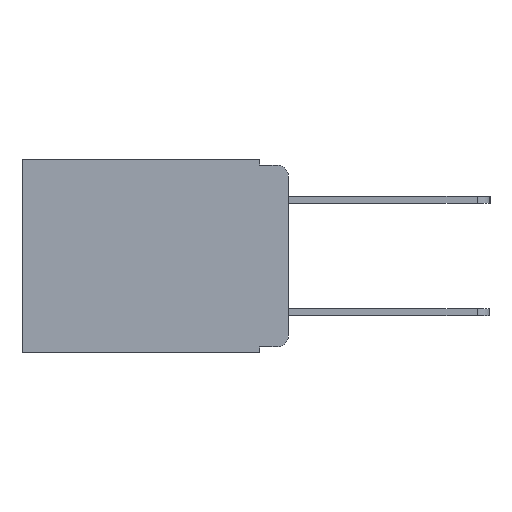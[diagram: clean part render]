
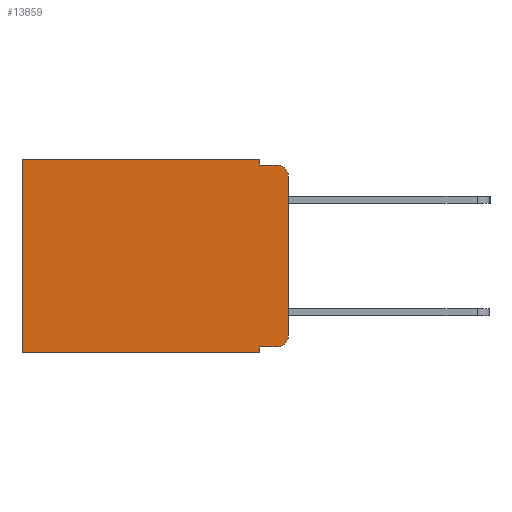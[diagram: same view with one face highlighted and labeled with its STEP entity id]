
A CAD part, left-side view. The second image highlights one B-rep face of the part: STEP entity #13859.
In plain terms, the highlighted planar face has unit normal (-1, 0, 0).
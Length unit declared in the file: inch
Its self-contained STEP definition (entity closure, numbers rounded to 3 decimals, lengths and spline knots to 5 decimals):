
#51 = CARTESIAN_POINT ( 'NONE',  ( 0.298, 0., -0.343 ) ) ;
#1154 = VECTOR ( 'NONE', #17467, 39.37008 ) ;
#1397 = EDGE_LOOP ( 'NONE', ( #1652, #6326, #1983, #3175, #3579, #5256, #9009, #4212, #4299, #4049 ) ) ;
#1432 = EDGE_CURVE ( 'NONE', #13218, #10000, #9390, .T. ) ;
#1652 = ORIENTED_EDGE ( 'NONE', *, *, #7734, .F. ) ;
#1961 = VECTOR ( 'NONE', #17110, 39.37008 ) ;
#1983 = ORIENTED_EDGE ( 'NONE', *, *, #1432, .F. ) ;
#2123 = VECTOR ( 'NONE', #3325, 39.37008 ) ;
#2561 = VECTOR ( 'NONE', #13670, 39.37008 ) ;
#2733 = CIRCLE ( 'NONE', #6456, 0.02 ) ;
#2882 = VECTOR ( 'NONE', #12268, 39.37008 ) ;
#2928 = CARTESIAN_POINT ( 'NONE',  ( 0.298, 0.051, 0. ) ) ;
#3175 = ORIENTED_EDGE ( 'NONE', *, *, #18427, .F. ) ;
#3248 = CARTESIAN_POINT ( 'NONE',  ( 0.298, 0.473, 0. ) ) ;
#3261 = PLANE ( 'NONE',  #17870 ) ;
#3325 = DIRECTION ( 'NONE',  ( 0., 0., -1. ) ) ;
#3501 = DIRECTION ( 'NONE',  ( 0., 0., -1. ) ) ;
#3526 = DIRECTION ( 'NONE',  ( -1., 0., 0. ) ) ;
#3579 = ORIENTED_EDGE ( 'NONE', *, *, #13932, .T. ) ;
#4049 = ORIENTED_EDGE ( 'NONE', *, *, #10074, .T. ) ;
#4212 = ORIENTED_EDGE ( 'NONE', *, *, #13877, .F. ) ;
#4299 = ORIENTED_EDGE ( 'NONE', *, *, #11007, .T. ) ;
#4329 = VERTEX_POINT ( 'NONE', #5411 ) ;
#4592 = EDGE_CURVE ( 'NONE', #17479, #10000, #2733, .T. ) ;
#4647 = CARTESIAN_POINT ( 'NONE',  ( 0.298, 0., -0.03 ) ) ;
#4791 = FACE_OUTER_BOUND ( 'NONE', #1397, .T. ) ;
#5071 = CARTESIAN_POINT ( 'NONE',  ( 0.298, 0.473, 0. ) ) ;
#5256 = ORIENTED_EDGE ( 'NONE', *, *, #15761, .T. ) ;
#5411 = CARTESIAN_POINT ( 'NONE',  ( 0.298, 0.051, -0.333 ) ) ;
#5616 = CARTESIAN_POINT ( 'NONE',  ( 0.298, 0.051, -0.333 ) ) ;
#6011 = CARTESIAN_POINT ( 'NONE',  ( 0.298, 0.02, -0.01 ) ) ;
#6326 = ORIENTED_EDGE ( 'NONE', *, *, #4592, .T. ) ;
#6417 = CARTESIAN_POINT ( 'NONE',  ( 0.298, 0.051, 0. ) ) ;
#6456 = AXIS2_PLACEMENT_3D ( 'NONE', #13480, #3526, #3501 ) ;
#6619 = LINE ( 'NONE', #5616, #1961 ) ;
#6720 = LINE ( 'NONE', #11252, #2561 ) ;
#7714 = CARTESIAN_POINT ( 'NONE',  ( 0.298, 0.051, -0.343 ) ) ;
#7734 = EDGE_CURVE ( 'NONE', #17479, #16970, #6720, .T. ) ;
#8359 = LINE ( 'NONE', #3248, #15492 ) ;
#8991 = LINE ( 'NONE', #2928, #9475 ) ;
#9009 = ORIENTED_EDGE ( 'NONE', *, *, #12259, .F. ) ;
#9024 = AXIS2_PLACEMENT_3D ( 'NONE', #17718, #9348, #9395 ) ;
#9348 = DIRECTION ( 'NONE',  ( -1., 0., 0. ) ) ;
#9390 = LINE ( 'NONE', #17449, #1154 ) ;
#9393 = CARTESIAN_POINT ( 'NONE',  ( 0.298, 0.473, -0.343 ) ) ;
#9395 = DIRECTION ( 'NONE',  ( 0., 0., -1. ) ) ;
#9453 = DIRECTION ( 'NONE',  ( 0., 0., -1. ) ) ;
#9475 = VECTOR ( 'NONE', #16165, 39.37008 ) ;
#10000 = VERTEX_POINT ( 'NONE', #6011 ) ;
#10074 = EDGE_CURVE ( 'NONE', #12933, #16970, #16953, .T. ) ;
#10734 = CARTESIAN_POINT ( 'NONE',  ( 0.298, 0.051, -0.01 ) ) ;
#10792 = DIRECTION ( 'NONE',  ( 0., 0., -1. ) ) ;
#10870 = CARTESIAN_POINT ( 'NONE',  ( 0.298, 0.051, 0. ) ) ;
#11007 = EDGE_CURVE ( 'NONE', #4329, #12933, #6619, .T. ) ;
#11205 = VERTEX_POINT ( 'NONE', #7714 ) ;
#11252 = CARTESIAN_POINT ( 'NONE',  ( 0.298, 0., 0. ) ) ;
#11333 = LINE ( 'NONE', #12441, #14664 ) ;
#12217 = LINE ( 'NONE', #10870, #2123 ) ;
#12237 = CARTESIAN_POINT ( 'NONE',  ( 0.298, 0., 0. ) ) ;
#12259 = EDGE_CURVE ( 'NONE', #11205, #15268, #18323, .T. ) ;
#12268 = DIRECTION ( 'NONE',  ( 0., 1., 0. ) ) ;
#12272 = CARTESIAN_POINT ( 'NONE',  ( 0.298, 0., -0.313 ) ) ;
#12441 = CARTESIAN_POINT ( 'NONE',  ( 0.298, 0., 0. ) ) ;
#12705 = VERTEX_POINT ( 'NONE', #5071 ) ;
#12933 = VERTEX_POINT ( 'NONE', #18438 ) ;
#13218 = VERTEX_POINT ( 'NONE', #10734 ) ;
#13480 = CARTESIAN_POINT ( 'NONE',  ( 0.298, 0.02, -0.03 ) ) ;
#13670 = DIRECTION ( 'NONE',  ( 0., 0., -1. ) ) ;
#13859 = ADVANCED_FACE ( 'NONE', ( #4791 ), #3261, .F. ) ;
#13877 = EDGE_CURVE ( 'NONE', #4329, #11205, #12217, .T. ) ;
#13932 = EDGE_CURVE ( 'NONE', #14355, #12705, #11333, .T. ) ;
#14355 = VERTEX_POINT ( 'NONE', #6417 ) ;
#14664 = VECTOR ( 'NONE', #15221, 39.37008 ) ;
#15221 = DIRECTION ( 'NONE',  ( 0., 1., 0. ) ) ;
#15268 = VERTEX_POINT ( 'NONE', #9393 ) ;
#15492 = VECTOR ( 'NONE', #10792, 39.37008 ) ;
#15761 = EDGE_CURVE ( 'NONE', #12705, #15268, #8359, .T. ) ;
#16165 = DIRECTION ( 'NONE',  ( 0., 0., -1. ) ) ;
#16953 = CIRCLE ( 'NONE', #9024, 0.02 ) ;
#16970 = VERTEX_POINT ( 'NONE', #12272 ) ;
#17110 = DIRECTION ( 'NONE',  ( 0., -1., 0. ) ) ;
#17449 = CARTESIAN_POINT ( 'NONE',  ( 0.298, 0.051, -0.01 ) ) ;
#17467 = DIRECTION ( 'NONE',  ( 0., -1., 0. ) ) ;
#17479 = VERTEX_POINT ( 'NONE', #4647 ) ;
#17718 = CARTESIAN_POINT ( 'NONE',  ( 0.298, 0.02, -0.313 ) ) ;
#17811 = DIRECTION ( 'NONE',  ( 1., 0., 0. ) ) ;
#17870 = AXIS2_PLACEMENT_3D ( 'NONE', #12237, #17811, #9453 ) ;
#18323 = LINE ( 'NONE', #51, #2882 ) ;
#18427 = EDGE_CURVE ( 'NONE', #14355, #13218, #8991, .T. ) ;
#18438 = CARTESIAN_POINT ( 'NONE',  ( 0.298, 0.02, -0.333 ) ) ;
